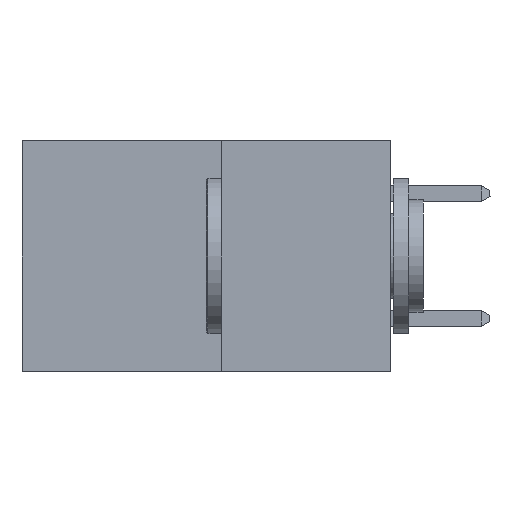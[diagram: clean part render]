
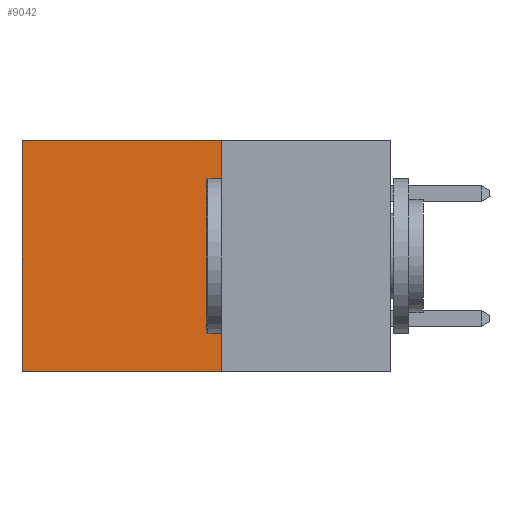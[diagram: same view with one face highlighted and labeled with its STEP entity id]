
A CAD part, left-side view. The second image highlights one B-rep face of the part: STEP entity #9042.
In plain terms, the highlighted planar face has unit normal (-1, 0, 0).
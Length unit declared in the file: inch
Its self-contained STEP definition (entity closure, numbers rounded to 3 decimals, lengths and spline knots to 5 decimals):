
#245 = DIRECTION ( 'NONE',  ( 0., 1., 0. ) ) ;
#422 = EDGE_CURVE ( 'NONE', #8432, #15596, #574, .T. ) ;
#574 = LINE ( 'NONE', #12650, #3608 ) ;
#924 = LINE ( 'NONE', #1583, #7354 ) ;
#1244 = LINE ( 'NONE', #4717, #14261 ) ;
#1347 = EDGE_CURVE ( 'NONE', #11710, #12509, #924, .T. ) ;
#1583 = CARTESIAN_POINT ( 'NONE',  ( 0.277, 0.27, -0.37 ) ) ;
#1730 = VECTOR ( 'NONE', #16006, 39.37008 ) ;
#2147 = LINE ( 'NONE', #6099, #1730 ) ;
#2641 = CARTESIAN_POINT ( 'NONE',  ( 0.277, 0.27, -0.37 ) ) ;
#3387 = ORIENTED_EDGE ( 'NONE', *, *, #11517, .F. ) ;
#3608 = VECTOR ( 'NONE', #13859, 39.37008 ) ;
#4649 = DIRECTION ( 'NONE',  ( 0., 0., -1. ) ) ;
#4717 = CARTESIAN_POINT ( 'NONE',  ( 0.277, 0.27, -0.37 ) ) ;
#6099 = CARTESIAN_POINT ( 'NONE',  ( 0.277, 0.59, -0.37 ) ) ;
#6376 = AXIS2_PLACEMENT_3D ( 'NONE', #15187, #15010, #14993 ) ;
#7354 = VECTOR ( 'NONE', #245, 39.37008 ) ;
#8219 = EDGE_LOOP ( 'NONE', ( #9324, #15880, #3387, #13393 ) ) ;
#8397 = CARTESIAN_POINT ( 'NONE',  ( 0.277, 0.27, 0. ) ) ;
#8432 = VERTEX_POINT ( 'NONE', #8397 ) ;
#9042 = ADVANCED_FACE ( 'NONE', ( #10523 ), #15028, .F. ) ;
#9324 = ORIENTED_EDGE ( 'NONE', *, *, #12718, .T. ) ;
#10523 = FACE_OUTER_BOUND ( 'NONE', #8219, .T. ) ;
#11517 = EDGE_CURVE ( 'NONE', #8432, #11710, #1244, .T. ) ;
#11710 = VERTEX_POINT ( 'NONE', #2641 ) ;
#11993 = CARTESIAN_POINT ( 'NONE',  ( 0.277, 0.59, 0. ) ) ;
#12509 = VERTEX_POINT ( 'NONE', #14421 ) ;
#12650 = CARTESIAN_POINT ( 'NONE',  ( 0.277, 0.27, 0. ) ) ;
#12718 = EDGE_CURVE ( 'NONE', #15596, #12509, #2147, .T. ) ;
#13393 = ORIENTED_EDGE ( 'NONE', *, *, #422, .T. ) ;
#13859 = DIRECTION ( 'NONE',  ( 0., 1., 0. ) ) ;
#14261 = VECTOR ( 'NONE', #4649, 39.37008 ) ;
#14421 = CARTESIAN_POINT ( 'NONE',  ( 0.277, 0.59, -0.37 ) ) ;
#14993 = DIRECTION ( 'NONE',  ( 0., 0., -1. ) ) ;
#15010 = DIRECTION ( 'NONE',  ( 1., 0., 0. ) ) ;
#15028 = PLANE ( 'NONE',  #6376 ) ;
#15187 = CARTESIAN_POINT ( 'NONE',  ( 0.277, 0.27, -0.37 ) ) ;
#15596 = VERTEX_POINT ( 'NONE', #11993 ) ;
#15880 = ORIENTED_EDGE ( 'NONE', *, *, #1347, .F. ) ;
#16006 = DIRECTION ( 'NONE',  ( 0., 0., -1. ) ) ;
